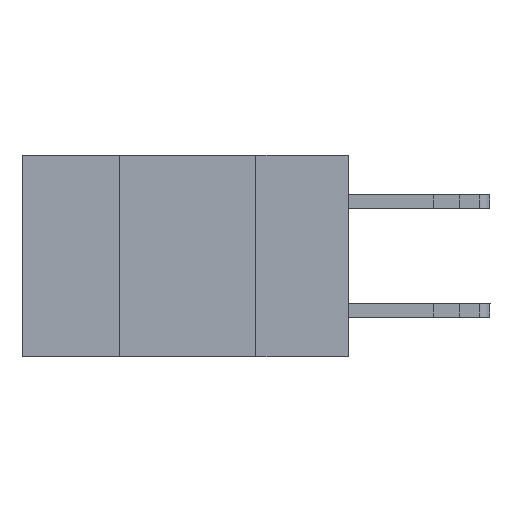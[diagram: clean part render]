
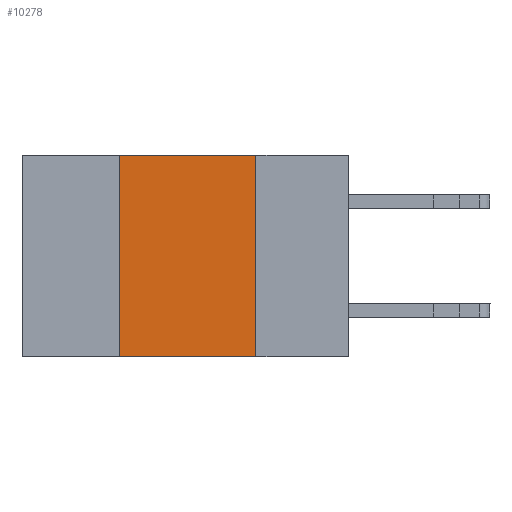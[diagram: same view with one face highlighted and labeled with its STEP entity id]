
A CAD part, left-side view. The second image highlights one B-rep face of the part: STEP entity #10278.
In plain terms, the highlighted planar face has unit normal (-1, 0, 0).
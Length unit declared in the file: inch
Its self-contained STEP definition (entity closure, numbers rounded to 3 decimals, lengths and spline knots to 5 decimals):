
#536 = DIRECTION ( 'NONE',  ( 0., -1., 0. ) ) ;
#1215 = EDGE_LOOP ( 'NONE', ( #16278, #14192, #10746, #9898 ) ) ;
#2456 = VECTOR ( 'NONE', #12206, 39.37008 ) ;
#3729 = EDGE_CURVE ( 'NONE', #16203, #9530, #6416, .T. ) ;
#3742 = DIRECTION ( 'NONE',  ( 0., 0., -1. ) ) ;
#3868 = VERTEX_POINT ( 'NONE', #11091 ) ;
#4597 = CARTESIAN_POINT ( 'NONE',  ( 0., 0.42, 0. ) ) ;
#6326 = VERTEX_POINT ( 'NONE', #7686 ) ;
#6416 = LINE ( 'NONE', #12280, #2456 ) ;
#6936 = LINE ( 'NONE', #13573, #10850 ) ;
#7284 = EDGE_CURVE ( 'NONE', #16203, #6326, #6936, .T. ) ;
#7686 = CARTESIAN_POINT ( 'NONE',  ( 0., 0.17, -0.37 ) ) ;
#7710 = VECTOR ( 'NONE', #3742, 39.37008 ) ;
#8502 = CARTESIAN_POINT ( 'NONE',  ( 0., 0.6, 0. ) ) ;
#9398 = VECTOR ( 'NONE', #536, 39.37008 ) ;
#9530 = VERTEX_POINT ( 'NONE', #4597 ) ;
#9898 = ORIENTED_EDGE ( 'NONE', *, *, #7284, .T. ) ;
#10278 = ADVANCED_FACE ( 'NONE', ( #16086 ), #10977, .F. ) ;
#10305 = CARTESIAN_POINT ( 'NONE',  ( 0., 0.17, -0.37 ) ) ;
#10746 = ORIENTED_EDGE ( 'NONE', *, *, #3729, .F. ) ;
#10794 = LINE ( 'NONE', #10305, #7710 ) ;
#10850 = VECTOR ( 'NONE', #13385, 39.37008 ) ;
#10940 = DIRECTION ( 'NONE',  ( 0., 0., -1. ) ) ;
#10963 = DIRECTION ( 'NONE',  ( 1., 0., 0. ) ) ;
#10977 = PLANE ( 'NONE',  #16914 ) ;
#11091 = CARTESIAN_POINT ( 'NONE',  ( 0., 0.17, 0. ) ) ;
#12013 = EDGE_CURVE ( 'NONE', #3868, #6326, #10794, .T. ) ;
#12206 = DIRECTION ( 'NONE',  ( 0., 0., 1. ) ) ;
#12280 = CARTESIAN_POINT ( 'NONE',  ( 0., 0.42, -0.37 ) ) ;
#13275 = LINE ( 'NONE', #8502, #9398 ) ;
#13385 = DIRECTION ( 'NONE',  ( 0., -1., 0. ) ) ;
#13573 = CARTESIAN_POINT ( 'NONE',  ( 0., 0.6, -0.37 ) ) ;
#13673 = CARTESIAN_POINT ( 'NONE',  ( 0., 0.6, 0. ) ) ;
#14192 = ORIENTED_EDGE ( 'NONE', *, *, #16593, .F. ) ;
#16086 = FACE_OUTER_BOUND ( 'NONE', #1215, .T. ) ;
#16203 = VERTEX_POINT ( 'NONE', #16742 ) ;
#16278 = ORIENTED_EDGE ( 'NONE', *, *, #12013, .F. ) ;
#16593 = EDGE_CURVE ( 'NONE', #9530, #3868, #13275, .T. ) ;
#16742 = CARTESIAN_POINT ( 'NONE',  ( 0., 0.42, -0.37 ) ) ;
#16914 = AXIS2_PLACEMENT_3D ( 'NONE', #13673, #10963, #10940 ) ;
